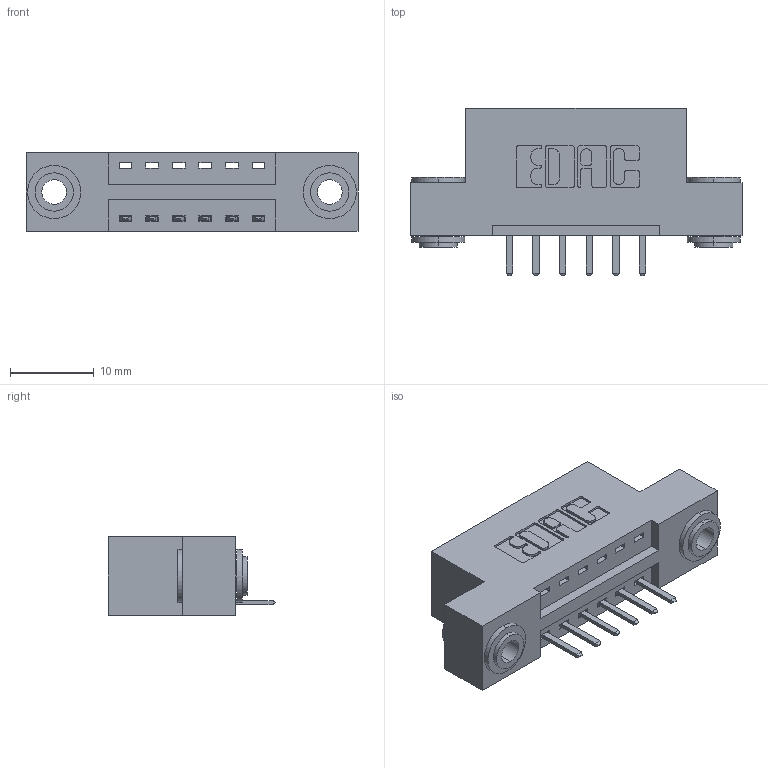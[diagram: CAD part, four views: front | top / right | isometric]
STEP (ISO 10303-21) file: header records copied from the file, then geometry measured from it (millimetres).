
FILE_DESCRIPTION (( 'STEP AP203' ), '1' );
FILE_NAME ('346-006-520-103.STEP', '2018-08-17T02:47:32', ( '' ), ( '' ), 'SwSTEP 2.0', 'SolidWorks 2016', '' );
FILE_SCHEMA (( 'CONFIG_CONTROL_DESIGN' ));
Length unit declared in the file: inch
Products named in the file (4): 346 Part_Flush Mounting Lugs - 0.156 Dia-TH; 345-292-001_345-293-120; 345-250-002_345-250-002-102; 346-006-520-103
Assembly tree (9 placements, depth 2):
  346-006-520-103
    346 Part_Flush Mounting Lugs - 0.156 Dia-TH
    345-292-001_345-293-120  x6
    345-250-002_345-250-002-102  x2
Bounding box: 39.62 x 20.02 x 9.4 mm (x, y, z)
Volume: 3547 mm3; surface area: 4206.4 mm2
Topology: 9 solids, 9 shells, 532 faces, 1509 edges, 986 vertices
Faces by surface type: plane 338, cylinder 186, cone 8
Entity records: 9334 total; most frequent: CARTESIAN_POINT 1601, ORIENTED_EDGE 1522, DIRECTION 1475, EDGE_CURVE 761, VECTOR 577, LINE 577, VERTEX_POINT 502, AXIS2_PLACEMENT_3D 449
